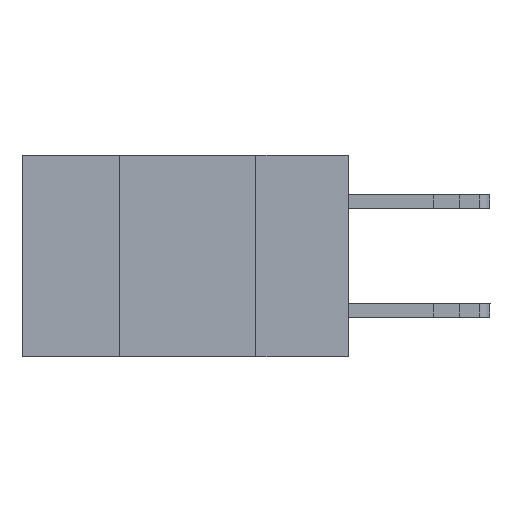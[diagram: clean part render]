
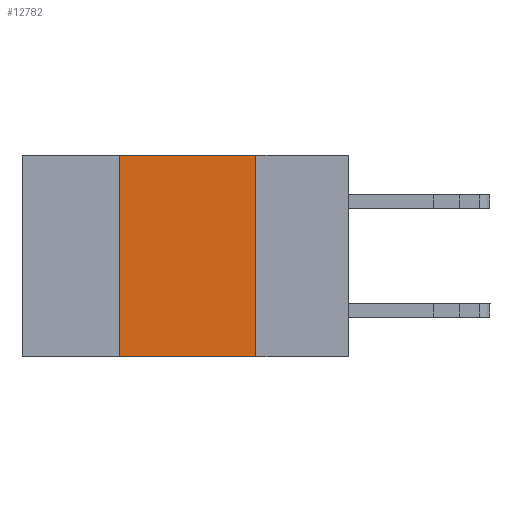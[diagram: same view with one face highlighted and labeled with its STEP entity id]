
A CAD part, left-side view. The second image highlights one B-rep face of the part: STEP entity #12782.
In plain terms, the highlighted planar face has unit normal (-1, 0, 0).
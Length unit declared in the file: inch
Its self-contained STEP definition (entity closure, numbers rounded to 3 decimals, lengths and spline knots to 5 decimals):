
#113 = AXIS2_PLACEMENT_3D ( 'NONE', #4587, #15052, #6099 ) ;
#376 = DIRECTION ( 'NONE',  ( 0., 0., 1. ) ) ;
#530 = DIRECTION ( 'NONE',  ( 0., 0., -1. ) ) ;
#1116 = EDGE_CURVE ( 'NONE', #13525, #17394, #16768, .T. ) ;
#1490 = EDGE_CURVE ( 'NONE', #10358, #14531, #18164, .T. ) ;
#2097 = LINE ( 'NONE', #2178, #17093 ) ;
#2178 = CARTESIAN_POINT ( 'NONE',  ( 0., 0.6, -0.37 ) ) ;
#3997 = CARTESIAN_POINT ( 'NONE',  ( 0., 0.6, 0. ) ) ;
#4587 = CARTESIAN_POINT ( 'NONE',  ( 0., 0.6, 0. ) ) ;
#4629 = CARTESIAN_POINT ( 'NONE',  ( 0., 0.17, -0.37 ) ) ;
#5009 = CARTESIAN_POINT ( 'NONE',  ( 0., 0.17, -0.37 ) ) ;
#5149 = DIRECTION ( 'NONE',  ( 0., -1., 0. ) ) ;
#6099 = DIRECTION ( 'NONE',  ( 0., 0., -1. ) ) ;
#8087 = CARTESIAN_POINT ( 'NONE',  ( 0., 0.42, 0. ) ) ;
#8895 = CARTESIAN_POINT ( 'NONE',  ( 0., 0.42, -0.37 ) ) ;
#9051 = EDGE_CURVE ( 'NONE', #17394, #10358, #17864, .T. ) ;
#9930 = VECTOR ( 'NONE', #18915, 39.37008 ) ;
#10204 = EDGE_CURVE ( 'NONE', #13525, #14531, #2097, .T. ) ;
#10358 = VERTEX_POINT ( 'NONE', #13008 ) ;
#10754 = EDGE_LOOP ( 'NONE', ( #13347, #11018, #17997, #16586 ) ) ;
#11018 = ORIENTED_EDGE ( 'NONE', *, *, #9051, .F. ) ;
#12064 = PLANE ( 'NONE',  #113 ) ;
#12782 = ADVANCED_FACE ( 'NONE', ( #14966 ), #12064, .F. ) ;
#12813 = VECTOR ( 'NONE', #376, 39.37008 ) ;
#13008 = CARTESIAN_POINT ( 'NONE',  ( 0., 0.17, 0. ) ) ;
#13347 = ORIENTED_EDGE ( 'NONE', *, *, #1490, .F. ) ;
#13525 = VERTEX_POINT ( 'NONE', #18178 ) ;
#14195 = VECTOR ( 'NONE', #530, 39.37008 ) ;
#14531 = VERTEX_POINT ( 'NONE', #4629 ) ;
#14966 = FACE_OUTER_BOUND ( 'NONE', #10754, .T. ) ;
#15052 = DIRECTION ( 'NONE',  ( 1., 0., 0. ) ) ;
#16586 = ORIENTED_EDGE ( 'NONE', *, *, #10204, .T. ) ;
#16768 = LINE ( 'NONE', #8895, #12813 ) ;
#17093 = VECTOR ( 'NONE', #5149, 39.37008 ) ;
#17394 = VERTEX_POINT ( 'NONE', #8087 ) ;
#17864 = LINE ( 'NONE', #3997, #9930 ) ;
#17997 = ORIENTED_EDGE ( 'NONE', *, *, #1116, .F. ) ;
#18164 = LINE ( 'NONE', #5009, #14195 ) ;
#18178 = CARTESIAN_POINT ( 'NONE',  ( 0., 0.42, -0.37 ) ) ;
#18915 = DIRECTION ( 'NONE',  ( 0., -1., 0. ) ) ;
